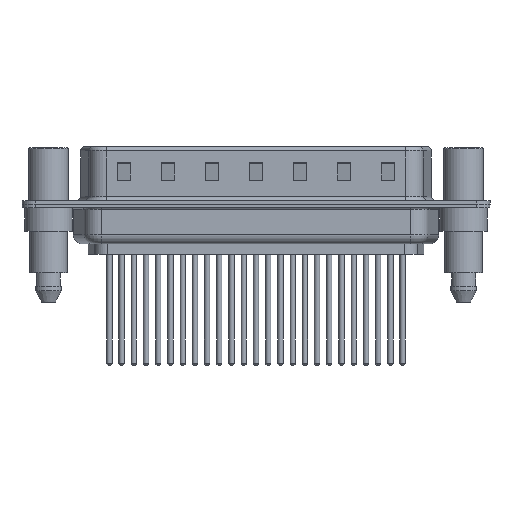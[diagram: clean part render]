
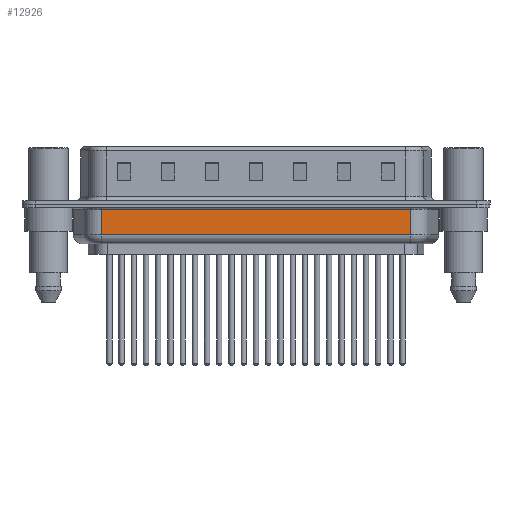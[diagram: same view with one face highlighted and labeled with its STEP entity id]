
A CAD part, front view. The second image highlights one B-rep face of the part: STEP entity #12926.
In plain terms, the highlighted planar face has unit normal (0, -1, 0).
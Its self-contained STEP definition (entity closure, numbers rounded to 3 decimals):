
#578 = EDGE_CURVE ( 'NONE', #3662, #2987, #18063, .T. ) ;
#659 = VERTEX_POINT ( 'NONE', #17960 ) ;
#1021 = CARTESIAN_POINT ( 'NONE',  ( 6.006, -5.35, -4.5 ) ) ;
#1145 = VECTOR ( 'NONE', #12404, 1000. ) ;
#2732 = DIRECTION ( 'NONE',  ( 0., 1., 0. ) ) ;
#2843 = FACE_OUTER_BOUND ( 'NONE', #14081, .T. ) ;
#2987 = VERTEX_POINT ( 'NONE', #10362 ) ;
#3018 = ORIENTED_EDGE ( 'NONE', *, *, #578, .T. ) ;
#3662 = VERTEX_POINT ( 'NONE', #12745 ) ;
#5734 = DIRECTION ( 'NONE',  ( 0., 0., 1. ) ) ;
#6287 = EDGE_CURVE ( 'NONE', #18118, #3662, #9169, .T. ) ;
#7302 = EDGE_CURVE ( 'NONE', #659, #2987, #8119, .T. ) ;
#8084 = DIRECTION ( 'NONE',  ( -1., 0., 0. ) ) ;
#8119 = LINE ( 'NONE', #14623, #1145 ) ;
#8792 = ORIENTED_EDGE ( 'NONE', *, *, #7302, .F. ) ;
#9169 = LINE ( 'NONE', #11475, #17607 ) ;
#9582 = CARTESIAN_POINT ( 'NONE',  ( 6.006, -5.35, -0.65 ) ) ;
#9758 = CARTESIAN_POINT ( 'NONE',  ( 6.006, -5.35, -3.5 ) ) ;
#10362 = CARTESIAN_POINT ( 'NONE',  ( 6.006, -5.35, -0.65 ) ) ;
#11281 = VECTOR ( 'NONE', #8084, 1000. ) ;
#11475 = CARTESIAN_POINT ( 'NONE',  ( 41.044, -5.35, -4.5 ) ) ;
#12033 = ORIENTED_EDGE ( 'NONE', *, *, #21077, .T. ) ;
#12404 = DIRECTION ( 'NONE',  ( 0., 0., 1. ) ) ;
#12617 = AXIS2_PLACEMENT_3D ( 'NONE', #1021, #2732, #5734 ) ;
#12745 = CARTESIAN_POINT ( 'NONE',  ( 41.044, -5.35, -0.65 ) ) ;
#12926 = ADVANCED_FACE ( 'NONE', ( #2843 ), #18949, .F. ) ;
#14081 = EDGE_LOOP ( 'NONE', ( #8792, #12033, #19293, #3018 ) ) ;
#14552 = LINE ( 'NONE', #9758, #14894 ) ;
#14623 = CARTESIAN_POINT ( 'NONE',  ( 6.006, -5.35, -4.5 ) ) ;
#14894 = VECTOR ( 'NONE', #21035, 1000. ) ;
#16819 = CARTESIAN_POINT ( 'NONE',  ( 41.044, -5.35, -3.5 ) ) ;
#17607 = VECTOR ( 'NONE', #18956, 1000. ) ;
#17960 = CARTESIAN_POINT ( 'NONE',  ( 6.006, -5.35, -3.5 ) ) ;
#18063 = LINE ( 'NONE', #9582, #11281 ) ;
#18118 = VERTEX_POINT ( 'NONE', #16819 ) ;
#18949 = PLANE ( 'NONE',  #12617 ) ;
#18956 = DIRECTION ( 'NONE',  ( 0., 0., 1. ) ) ;
#19293 = ORIENTED_EDGE ( 'NONE', *, *, #6287, .T. ) ;
#21035 = DIRECTION ( 'NONE',  ( 1., 0., 0. ) ) ;
#21077 = EDGE_CURVE ( 'NONE', #659, #18118, #14552, .T. ) ;
